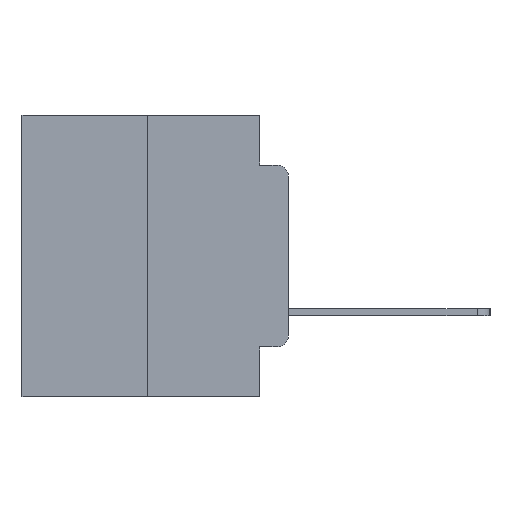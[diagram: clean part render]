
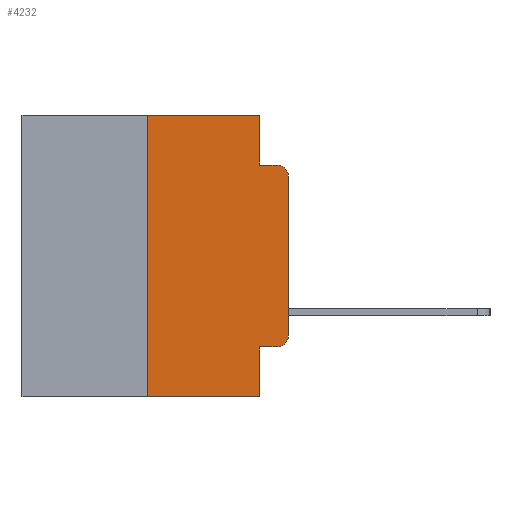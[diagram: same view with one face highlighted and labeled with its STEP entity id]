
A CAD part, left-side view. The second image highlights one B-rep face of the part: STEP entity #4232.
In plain terms, the highlighted planar face has unit normal (-1, 0, 0).
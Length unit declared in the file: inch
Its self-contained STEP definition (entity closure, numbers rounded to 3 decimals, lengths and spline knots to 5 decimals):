
#571 = VECTOR ( 'NONE', #8288, 39.37008 ) ;
#752 = VECTOR ( 'NONE', #15319, 39.37008 ) ;
#845 = CIRCLE ( 'NONE', #20495, 0.02 ) ;
#985 = CARTESIAN_POINT ( 'NONE',  ( 0., 0.051, 0. ) ) ;
#1018 = ORIENTED_EDGE ( 'NONE', *, *, #6770, .F. ) ;
#1497 = CARTESIAN_POINT ( 'NONE',  ( 0., 0.473, 0. ) ) ;
#1571 = CARTESIAN_POINT ( 'NONE',  ( 0., 0.02, -0.4115 ) ) ;
#1593 = DIRECTION ( 'NONE',  ( -1., 0., 0. ) ) ;
#2400 = EDGE_CURVE ( 'NONE', #25256, #20524, #12599, .T. ) ;
#3315 = DIRECTION ( 'NONE',  ( 1., 0., 0. ) ) ;
#4232 = ADVANCED_FACE ( 'NONE', ( #12090 ), #5501, .F. ) ;
#4276 = LINE ( 'NONE', #1497, #24536 ) ;
#4458 = VERTEX_POINT ( 'NONE', #20986 ) ;
#4844 = ORIENTED_EDGE ( 'NONE', *, *, #12161, .T. ) ;
#5336 = EDGE_CURVE ( 'NONE', #25256, #15535, #15766, .T. ) ;
#5501 = PLANE ( 'NONE',  #9496 ) ;
#5704 = VECTOR ( 'NONE', #23140, 39.37008 ) ;
#6228 = CARTESIAN_POINT ( 'NONE',  ( 0., 0., -0.1085 ) ) ;
#6359 = CARTESIAN_POINT ( 'NONE',  ( 0., 0.02, -0.0885 ) ) ;
#6402 = LINE ( 'NONE', #9706, #5704 ) ;
#6457 = LINE ( 'NONE', #16151, #571 ) ;
#6769 = DIRECTION ( 'NONE',  ( -1., 0., 0. ) ) ;
#6770 = EDGE_CURVE ( 'NONE', #23823, #25734, #21937, .T. ) ;
#6813 = EDGE_CURVE ( 'NONE', #25734, #14419, #4276, .T. ) ;
#7211 = VERTEX_POINT ( 'NONE', #12020 ) ;
#7340 = VERTEX_POINT ( 'NONE', #6359 ) ;
#7492 = CARTESIAN_POINT ( 'NONE',  ( 0., 0.051, -0.4115 ) ) ;
#7736 = CARTESIAN_POINT ( 'NONE',  ( 0., 0.473, -0.5 ) ) ;
#8179 = CARTESIAN_POINT ( 'NONE',  ( 0., 0.25, -0.5 ) ) ;
#8207 = EDGE_CURVE ( 'NONE', #14419, #4458, #6457, .T. ) ;
#8288 = DIRECTION ( 'NONE',  ( 0., 0., -1. ) ) ;
#9478 = ORIENTED_EDGE ( 'NONE', *, *, #2400, .T. ) ;
#9496 = AXIS2_PLACEMENT_3D ( 'NONE', #21279, #3315, #17291 ) ;
#9572 = EDGE_CURVE ( 'NONE', #4458, #7340, #24353, .T. ) ;
#9706 = CARTESIAN_POINT ( 'NONE',  ( 0., 0., 0. ) ) ;
#10515 = VECTOR ( 'NONE', #21206, 39.37008 ) ;
#10862 = EDGE_CURVE ( 'NONE', #24187, #7340, #14670, .T. ) ;
#11002 = EDGE_LOOP ( 'NONE', ( #4844, #15623, #20641, #11584, #21838, #1018, #12816, #18067, #9478, #25322 ) ) ;
#11584 = ORIENTED_EDGE ( 'NONE', *, *, #8207, .F. ) ;
#12020 = CARTESIAN_POINT ( 'NONE',  ( 0., 0., -0.3915 ) ) ;
#12090 = FACE_OUTER_BOUND ( 'NONE', #11002, .T. ) ;
#12161 = EDGE_CURVE ( 'NONE', #7211, #24187, #6402, .T. ) ;
#12599 = LINE ( 'NONE', #24676, #752 ) ;
#12816 = ORIENTED_EDGE ( 'NONE', *, *, #19037, .T. ) ;
#14057 = CARTESIAN_POINT ( 'NONE',  ( 0., 0.02, -0.3915 ) ) ;
#14306 = VECTOR ( 'NONE', #18843, 39.37008 ) ;
#14392 = CARTESIAN_POINT ( 'NONE',  ( 0., 0.051, -0.5 ) ) ;
#14419 = VERTEX_POINT ( 'NONE', #18144 ) ;
#14670 = CIRCLE ( 'NONE', #15081, 0.02 ) ;
#14811 = LINE ( 'NONE', #7736, #19295 ) ;
#15081 = AXIS2_PLACEMENT_3D ( 'NONE', #18641, #6769, #20494 ) ;
#15319 = DIRECTION ( 'NONE',  ( 0., -1., 0. ) ) ;
#15535 = VERTEX_POINT ( 'NONE', #14392 ) ;
#15623 = ORIENTED_EDGE ( 'NONE', *, *, #10862, .T. ) ;
#15766 = LINE ( 'NONE', #985, #10515 ) ;
#16016 = DIRECTION ( 'NONE',  ( 0., 0., -1. ) ) ;
#16151 = CARTESIAN_POINT ( 'NONE',  ( 0., 0.051, 0. ) ) ;
#16942 = CARTESIAN_POINT ( 'NONE',  ( 0., 0.051, -0.0885 ) ) ;
#17291 = DIRECTION ( 'NONE',  ( 0., 0., -1. ) ) ;
#18067 = ORIENTED_EDGE ( 'NONE', *, *, #5336, .F. ) ;
#18144 = CARTESIAN_POINT ( 'NONE',  ( 0., 0.051, 0. ) ) ;
#18641 = CARTESIAN_POINT ( 'NONE',  ( 0., 0.02, -0.1085 ) ) ;
#18843 = DIRECTION ( 'NONE',  ( 0., -1., 0. ) ) ;
#19037 = EDGE_CURVE ( 'NONE', #23823, #15535, #14811, .T. ) ;
#19295 = VECTOR ( 'NONE', #23235, 39.37008 ) ;
#20494 = DIRECTION ( 'NONE',  ( 0., 0., -1. ) ) ;
#20495 = AXIS2_PLACEMENT_3D ( 'NONE', #14057, #1593, #16016 ) ;
#20524 = VERTEX_POINT ( 'NONE', #1571 ) ;
#20641 = ORIENTED_EDGE ( 'NONE', *, *, #9572, .F. ) ;
#20986 = CARTESIAN_POINT ( 'NONE',  ( 0., 0.051, -0.0885 ) ) ;
#21206 = DIRECTION ( 'NONE',  ( 0., 0., -1. ) ) ;
#21279 = CARTESIAN_POINT ( 'NONE',  ( 0., 0.473, 0. ) ) ;
#21331 = VECTOR ( 'NONE', #25204, 39.37008 ) ;
#21384 = CARTESIAN_POINT ( 'NONE',  ( 0., 0.25, 0. ) ) ;
#21838 = ORIENTED_EDGE ( 'NONE', *, *, #6813, .F. ) ;
#21937 = LINE ( 'NONE', #21384, #21331 ) ;
#23140 = DIRECTION ( 'NONE',  ( 0., 0., 1. ) ) ;
#23235 = DIRECTION ( 'NONE',  ( 0., -1., 0. ) ) ;
#23823 = VERTEX_POINT ( 'NONE', #8179 ) ;
#24187 = VERTEX_POINT ( 'NONE', #6228 ) ;
#24353 = LINE ( 'NONE', #16942, #14306 ) ;
#24536 = VECTOR ( 'NONE', #25355, 39.37008 ) ;
#24676 = CARTESIAN_POINT ( 'NONE',  ( 0., 0.051, -0.4115 ) ) ;
#25204 = DIRECTION ( 'NONE',  ( 0., 0., 1. ) ) ;
#25256 = VERTEX_POINT ( 'NONE', #7492 ) ;
#25322 = ORIENTED_EDGE ( 'NONE', *, *, #25411, .T. ) ;
#25355 = DIRECTION ( 'NONE',  ( 0., -1., 0. ) ) ;
#25411 = EDGE_CURVE ( 'NONE', #20524, #7211, #845, .T. ) ;
#25527 = CARTESIAN_POINT ( 'NONE',  ( 0., 0.25, 0. ) ) ;
#25734 = VERTEX_POINT ( 'NONE', #25527 ) ;
